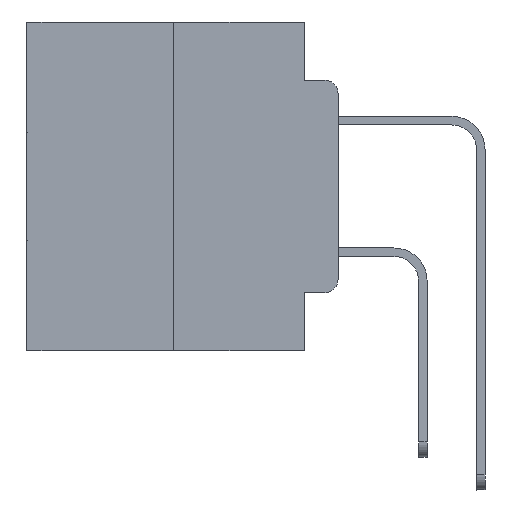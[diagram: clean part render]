
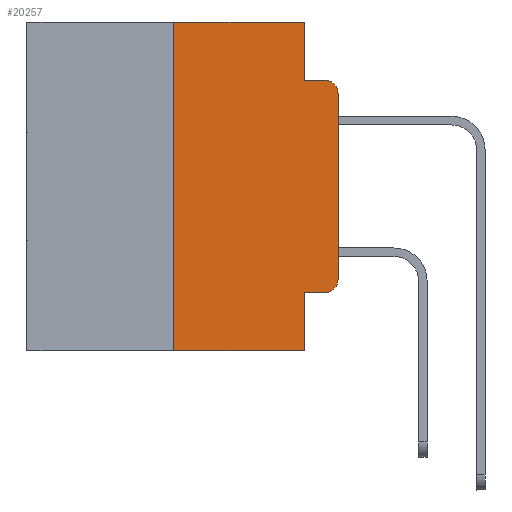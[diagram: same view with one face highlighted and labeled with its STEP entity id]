
A CAD part, left-side view. The second image highlights one B-rep face of the part: STEP entity #20257.
In plain terms, the highlighted planar face has unit normal (-1, 0, 0).
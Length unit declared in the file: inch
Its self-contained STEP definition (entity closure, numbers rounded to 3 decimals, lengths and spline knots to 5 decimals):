
#28 = DIRECTION ( 'NONE',  ( 0., 0., -1. ) ) ;
#380 = CARTESIAN_POINT ( 'NONE',  ( 0., 0.25, 0. ) ) ;
#483 = DIRECTION ( 'NONE',  ( 0., 0., 1. ) ) ;
#802 = EDGE_CURVE ( 'NONE', #23317, #17699, #22786, .T. ) ;
#1337 = CARTESIAN_POINT ( 'NONE',  ( 0., 0.02, -0.0885 ) ) ;
#1865 = ORIENTED_EDGE ( 'NONE', *, *, #19045, .F. ) ;
#2122 = VERTEX_POINT ( 'NONE', #12501 ) ;
#2442 = VECTOR ( 'NONE', #27760, 39.37008 ) ;
#3645 = LINE ( 'NONE', #29199, #27090 ) ;
#3920 = VECTOR ( 'NONE', #23340, 39.37008 ) ;
#3945 = VERTEX_POINT ( 'NONE', #23209 ) ;
#4475 = CARTESIAN_POINT ( 'NONE',  ( 0., 0., 0. ) ) ;
#5144 = EDGE_CURVE ( 'NONE', #16933, #11237, #28098, .T. ) ;
#5227 = EDGE_CURVE ( 'NONE', #23317, #15920, #19987, .T. ) ;
#5264 = DIRECTION ( 'NONE',  ( 1., 0., 0. ) ) ;
#5275 = CARTESIAN_POINT ( 'NONE',  ( 0., 0., -0.1085 ) ) ;
#5288 = VECTOR ( 'NONE', #26986, 39.37008 ) ;
#5617 = CARTESIAN_POINT ( 'NONE',  ( 0., 0.051, -0.0885 ) ) ;
#6026 = CIRCLE ( 'NONE', #16961, 0.02 ) ;
#6165 = VECTOR ( 'NONE', #483, 39.37008 ) ;
#6185 = EDGE_CURVE ( 'NONE', #7716, #2122, #18552, .T. ) ;
#6477 = CARTESIAN_POINT ( 'NONE',  ( 0., 0.25, -0.5 ) ) ;
#6737 = DIRECTION ( 'NONE',  ( -1., 0., 0. ) ) ;
#6825 = DIRECTION ( 'NONE',  ( 0., 0., 1. ) ) ;
#6950 = CARTESIAN_POINT ( 'NONE',  ( 0., 0.051, -0.4115 ) ) ;
#7419 = CARTESIAN_POINT ( 'NONE',  ( 0., 0.473, 0. ) ) ;
#7716 = VERTEX_POINT ( 'NONE', #26702 ) ;
#8139 = ORIENTED_EDGE ( 'NONE', *, *, #21186, .T. ) ;
#8790 = LINE ( 'NONE', #4475, #19391 ) ;
#9528 = EDGE_CURVE ( 'NONE', #3945, #16933, #8790, .T. ) ;
#11237 = VERTEX_POINT ( 'NONE', #1337 ) ;
#11434 = LINE ( 'NONE', #20202, #5288 ) ;
#12501 = CARTESIAN_POINT ( 'NONE',  ( 0., 0.051, 0. ) ) ;
#12569 = VECTOR ( 'NONE', #12979, 39.37008 ) ;
#12780 = ORIENTED_EDGE ( 'NONE', *, *, #17365, .F. ) ;
#12883 = CARTESIAN_POINT ( 'NONE',  ( 0., 0.473, 0. ) ) ;
#12915 = FACE_OUTER_BOUND ( 'NONE', #19329, .T. ) ;
#12979 = DIRECTION ( 'NONE',  ( 0., -1., 0. ) ) ;
#14010 = DIRECTION ( 'NONE',  ( -1., 0., 0. ) ) ;
#14218 = VECTOR ( 'NONE', #28285, 39.37008 ) ;
#14306 = CARTESIAN_POINT ( 'NONE',  ( 0., 0.051, -0.4115 ) ) ;
#14401 = PLANE ( 'NONE',  #15608 ) ;
#15095 = VERTEX_POINT ( 'NONE', #28231 ) ;
#15608 = AXIS2_PLACEMENT_3D ( 'NONE', #7419, #5264, #21142 ) ;
#15920 = VERTEX_POINT ( 'NONE', #23993 ) ;
#16374 = EDGE_CURVE ( 'NONE', #15095, #11237, #20160, .T. ) ;
#16933 = VERTEX_POINT ( 'NONE', #5275 ) ;
#16961 = AXIS2_PLACEMENT_3D ( 'NONE', #20293, #6737, #22559 ) ;
#17365 = EDGE_CURVE ( 'NONE', #2122, #15095, #3645, .T. ) ;
#17699 = VERTEX_POINT ( 'NONE', #23597 ) ;
#18270 = LINE ( 'NONE', #380, #6165 ) ;
#18552 = LINE ( 'NONE', #12883, #12569 ) ;
#18764 = ORIENTED_EDGE ( 'NONE', *, *, #6185, .F. ) ;
#19045 = EDGE_CURVE ( 'NONE', #22417, #7716, #18270, .T. ) ;
#19329 = EDGE_LOOP ( 'NONE', ( #27890, #28599, #23320, #12780, #18764, #1865, #8139, #20842, #26825, #21553 ) ) ;
#19391 = VECTOR ( 'NONE', #6825, 39.37008 ) ;
#19987 = LINE ( 'NONE', #14306, #2442 ) ;
#20160 = LINE ( 'NONE', #5617, #14218 ) ;
#20202 = CARTESIAN_POINT ( 'NONE',  ( 0., 0.473, -0.5 ) ) ;
#20257 = ADVANCED_FACE ( 'NONE', ( #12915 ), #14401, .F. ) ;
#20293 = CARTESIAN_POINT ( 'NONE',  ( 0., 0.02, -0.3915 ) ) ;
#20842 = ORIENTED_EDGE ( 'NONE', *, *, #802, .F. ) ;
#21142 = DIRECTION ( 'NONE',  ( 0., 0., -1. ) ) ;
#21186 = EDGE_CURVE ( 'NONE', #22417, #17699, #11434, .T. ) ;
#21194 = EDGE_CURVE ( 'NONE', #15920, #3945, #6026, .T. ) ;
#21553 = ORIENTED_EDGE ( 'NONE', *, *, #21194, .T. ) ;
#22417 = VERTEX_POINT ( 'NONE', #6477 ) ;
#22559 = DIRECTION ( 'NONE',  ( 0., 0., -1. ) ) ;
#22786 = LINE ( 'NONE', #23284, #3920 ) ;
#23209 = CARTESIAN_POINT ( 'NONE',  ( 0., 0., -0.3915 ) ) ;
#23284 = CARTESIAN_POINT ( 'NONE',  ( 0., 0.051, 0. ) ) ;
#23317 = VERTEX_POINT ( 'NONE', #6950 ) ;
#23320 = ORIENTED_EDGE ( 'NONE', *, *, #16374, .F. ) ;
#23340 = DIRECTION ( 'NONE',  ( 0., 0., -1. ) ) ;
#23597 = CARTESIAN_POINT ( 'NONE',  ( 0., 0.051, -0.5 ) ) ;
#23993 = CARTESIAN_POINT ( 'NONE',  ( 0., 0.02, -0.4115 ) ) ;
#24776 = DIRECTION ( 'NONE',  ( 0., 0., -1. ) ) ;
#26702 = CARTESIAN_POINT ( 'NONE',  ( 0., 0.25, 0. ) ) ;
#26825 = ORIENTED_EDGE ( 'NONE', *, *, #5227, .T. ) ;
#26986 = DIRECTION ( 'NONE',  ( 0., -1., 0. ) ) ;
#27090 = VECTOR ( 'NONE', #24776, 39.37008 ) ;
#27470 = CARTESIAN_POINT ( 'NONE',  ( 0., 0.02, -0.1085 ) ) ;
#27760 = DIRECTION ( 'NONE',  ( 0., -1., 0. ) ) ;
#27890 = ORIENTED_EDGE ( 'NONE', *, *, #9528, .T. ) ;
#28098 = CIRCLE ( 'NONE', #28141, 0.02 ) ;
#28141 = AXIS2_PLACEMENT_3D ( 'NONE', #27470, #14010, #28 ) ;
#28231 = CARTESIAN_POINT ( 'NONE',  ( 0., 0.051, -0.0885 ) ) ;
#28285 = DIRECTION ( 'NONE',  ( 0., -1., 0. ) ) ;
#28599 = ORIENTED_EDGE ( 'NONE', *, *, #5144, .T. ) ;
#29199 = CARTESIAN_POINT ( 'NONE',  ( 0., 0.051, 0. ) ) ;
